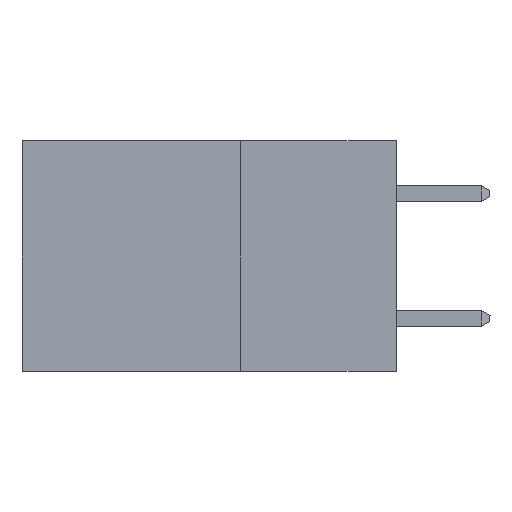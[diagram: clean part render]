
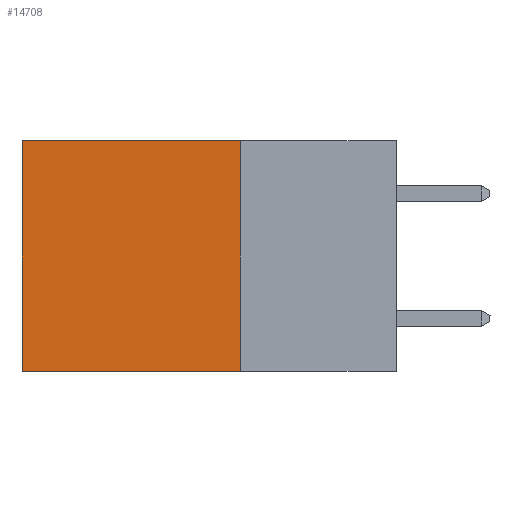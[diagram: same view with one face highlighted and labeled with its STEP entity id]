
A CAD part, left-side view. The second image highlights one B-rep face of the part: STEP entity #14708.
In plain terms, the highlighted planar face has unit normal (-1, 0, 0).
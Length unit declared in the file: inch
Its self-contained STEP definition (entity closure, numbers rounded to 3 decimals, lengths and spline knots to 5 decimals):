
#861 = VECTOR ( 'NONE', #4765, 39.37008 ) ;
#899 = CARTESIAN_POINT ( 'NONE',  ( 0.2615, 0.25, -0.37 ) ) ;
#917 = PLANE ( 'NONE',  #14097 ) ;
#1095 = LINE ( 'NONE', #10826, #4824 ) ;
#1287 = EDGE_LOOP ( 'NONE', ( #18789, #18564, #2469, #15969 ) ) ;
#1586 = CARTESIAN_POINT ( 'NONE',  ( 0.2615, 0.6, -0.37 ) ) ;
#1891 = VERTEX_POINT ( 'NONE', #12121 ) ;
#2469 = ORIENTED_EDGE ( 'NONE', *, *, #12563, .F. ) ;
#2522 = DIRECTION ( 'NONE',  ( 0., 1., 0. ) ) ;
#4134 = DIRECTION ( 'NONE',  ( 0., 0., -1. ) ) ;
#4444 = CARTESIAN_POINT ( 'NONE',  ( 0.2615, 0.25, 0. ) ) ;
#4765 = DIRECTION ( 'NONE',  ( 0., 0., -1. ) ) ;
#4824 = VECTOR ( 'NONE', #12439, 39.37008 ) ;
#6911 = CARTESIAN_POINT ( 'NONE',  ( 0.2615, 0.25, -0.37 ) ) ;
#8869 = CARTESIAN_POINT ( 'NONE',  ( 0.2615, 0.6, -0.37 ) ) ;
#9147 = CARTESIAN_POINT ( 'NONE',  ( 0.2615, 0.25, -0.37 ) ) ;
#10109 = DIRECTION ( 'NONE',  ( 0., 0., -1. ) ) ;
#10826 = CARTESIAN_POINT ( 'NONE',  ( 0.2615, 0.25, 0. ) ) ;
#11798 = LINE ( 'NONE', #6911, #20235 ) ;
#11997 = CARTESIAN_POINT ( 'NONE',  ( 0.2615, 0.25, -0.37 ) ) ;
#12121 = CARTESIAN_POINT ( 'NONE',  ( 0.2615, 0.6, 0. ) ) ;
#12439 = DIRECTION ( 'NONE',  ( 0., 1., 0. ) ) ;
#12563 = EDGE_CURVE ( 'NONE', #15819, #16529, #11798, .T. ) ;
#13550 = LINE ( 'NONE', #1586, #861 ) ;
#13629 = DIRECTION ( 'NONE',  ( 1., 0., 0. ) ) ;
#13658 = EDGE_CURVE ( 'NONE', #1891, #18313, #13550, .T. ) ;
#14097 = AXIS2_PLACEMENT_3D ( 'NONE', #11997, #13629, #4134 ) ;
#14211 = LINE ( 'NONE', #899, #17956 ) ;
#14708 = ADVANCED_FACE ( 'NONE', ( #19439 ), #917, .F. ) ;
#15617 = EDGE_CURVE ( 'NONE', #16529, #18313, #14211, .T. ) ;
#15819 = VERTEX_POINT ( 'NONE', #4444 ) ;
#15969 = ORIENTED_EDGE ( 'NONE', *, *, #16558, .T. ) ;
#16529 = VERTEX_POINT ( 'NONE', #9147 ) ;
#16558 = EDGE_CURVE ( 'NONE', #15819, #1891, #1095, .T. ) ;
#17956 = VECTOR ( 'NONE', #2522, 39.37008 ) ;
#18313 = VERTEX_POINT ( 'NONE', #8869 ) ;
#18564 = ORIENTED_EDGE ( 'NONE', *, *, #15617, .F. ) ;
#18789 = ORIENTED_EDGE ( 'NONE', *, *, #13658, .T. ) ;
#19439 = FACE_OUTER_BOUND ( 'NONE', #1287, .T. ) ;
#20235 = VECTOR ( 'NONE', #10109, 39.37008 ) ;
